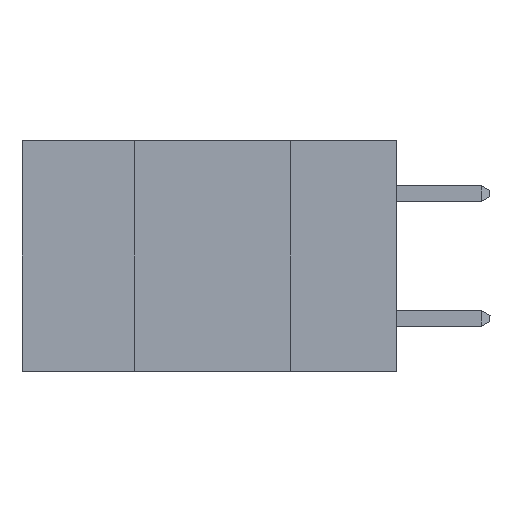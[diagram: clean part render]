
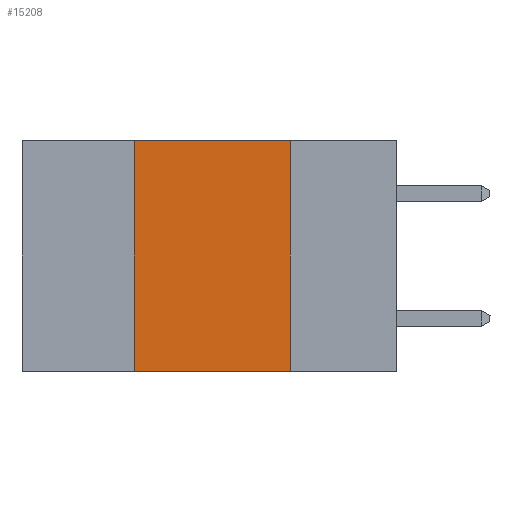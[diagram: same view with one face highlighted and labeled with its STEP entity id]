
A CAD part, left-side view. The second image highlights one B-rep face of the part: STEP entity #15208.
In plain terms, the highlighted planar face has unit normal (-1, 0, 0).
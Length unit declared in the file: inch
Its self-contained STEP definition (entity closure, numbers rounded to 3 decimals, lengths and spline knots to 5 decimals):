
#67 = CARTESIAN_POINT ( 'NONE',  ( 0., 0.42, 0. ) ) ;
#603 = VERTEX_POINT ( 'NONE', #6805 ) ;
#866 = VECTOR ( 'NONE', #12773, 39.37008 ) ;
#1227 = DIRECTION ( 'NONE',  ( 0., 0., 1. ) ) ;
#1456 = LINE ( 'NONE', #3778, #866 ) ;
#2074 = ORIENTED_EDGE ( 'NONE', *, *, #10850, .F. ) ;
#2931 = EDGE_LOOP ( 'NONE', ( #15081, #9698, #2074, #12648 ) ) ;
#3378 = CARTESIAN_POINT ( 'NONE',  ( 0., 0.17, 0. ) ) ;
#3451 = EDGE_CURVE ( 'NONE', #15415, #603, #1456, .T. ) ;
#3778 = CARTESIAN_POINT ( 'NONE',  ( 0., 0.6, -0.37 ) ) ;
#4845 = VECTOR ( 'NONE', #12387, 39.37008 ) ;
#5335 = FACE_OUTER_BOUND ( 'NONE', #2931, .T. ) ;
#5611 = PLANE ( 'NONE',  #11763 ) ;
#6304 = EDGE_CURVE ( 'NONE', #11801, #11471, #9176, .T. ) ;
#6805 = CARTESIAN_POINT ( 'NONE',  ( 0., 0.17, -0.37 ) ) ;
#7374 = VECTOR ( 'NONE', #15191, 39.37008 ) ;
#8235 = CARTESIAN_POINT ( 'NONE',  ( 0., 0.6, 0. ) ) ;
#8450 = DIRECTION ( 'NONE',  ( 0., 0., -1. ) ) ;
#9176 = LINE ( 'NONE', #10918, #7374 ) ;
#9698 = ORIENTED_EDGE ( 'NONE', *, *, #6304, .F. ) ;
#10200 = EDGE_CURVE ( 'NONE', #11471, #603, #12906, .T. ) ;
#10232 = CARTESIAN_POINT ( 'NONE',  ( 0., 0.17, 0. ) ) ;
#10850 = EDGE_CURVE ( 'NONE', #15415, #11801, #11274, .T. ) ;
#10874 = VECTOR ( 'NONE', #1227, 39.37008 ) ;
#10918 = CARTESIAN_POINT ( 'NONE',  ( 0., 0.6, 0. ) ) ;
#10986 = CARTESIAN_POINT ( 'NONE',  ( 0., 0.42, 0. ) ) ;
#11274 = LINE ( 'NONE', #67, #10874 ) ;
#11471 = VERTEX_POINT ( 'NONE', #10232 ) ;
#11763 = AXIS2_PLACEMENT_3D ( 'NONE', #8235, #14790, #8450 ) ;
#11801 = VERTEX_POINT ( 'NONE', #10986 ) ;
#11814 = CARTESIAN_POINT ( 'NONE',  ( 0., 0.42, -0.37 ) ) ;
#12387 = DIRECTION ( 'NONE',  ( 0., 0., -1. ) ) ;
#12648 = ORIENTED_EDGE ( 'NONE', *, *, #3451, .T. ) ;
#12773 = DIRECTION ( 'NONE',  ( 0., -1., 0. ) ) ;
#12906 = LINE ( 'NONE', #3378, #4845 ) ;
#14790 = DIRECTION ( 'NONE',  ( 1., 0., 0. ) ) ;
#15081 = ORIENTED_EDGE ( 'NONE', *, *, #10200, .F. ) ;
#15191 = DIRECTION ( 'NONE',  ( 0., -1., 0. ) ) ;
#15208 = ADVANCED_FACE ( 'NONE', ( #5335 ), #5611, .F. ) ;
#15415 = VERTEX_POINT ( 'NONE', #11814 ) ;
